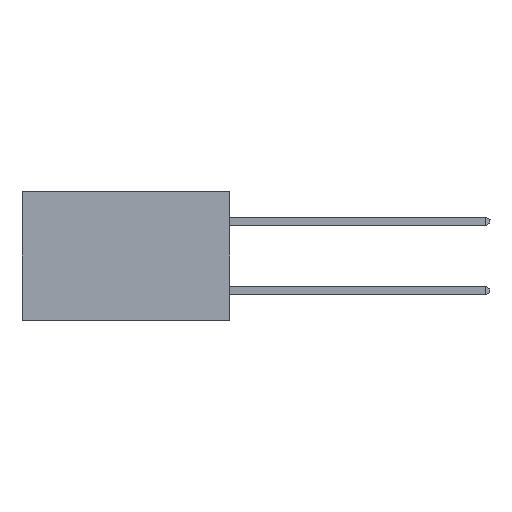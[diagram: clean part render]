
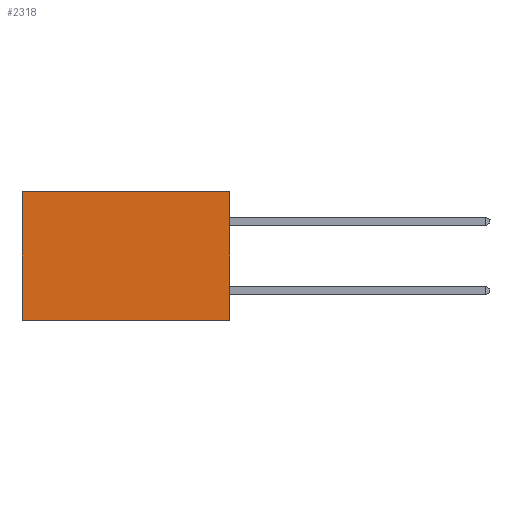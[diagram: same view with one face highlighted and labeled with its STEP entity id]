
A CAD part, left-side view. The second image highlights one B-rep face of the part: STEP entity #2318.
In plain terms, the highlighted planar face has unit normal (-1, 0, 0).
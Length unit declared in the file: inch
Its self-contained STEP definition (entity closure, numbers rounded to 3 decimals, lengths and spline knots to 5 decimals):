
#1065 = LINE ( 'NONE', #1849, #16956 ) ;
#1780 = EDGE_CURVE ( 'NONE', #18453, #9391, #6993, .T. ) ;
#1849 = CARTESIAN_POINT ( 'NONE',  ( 0.298, 0., 0. ) ) ;
#2318 = ADVANCED_FACE ( 'NONE', ( #10738 ), #8810, .F. ) ;
#3402 = CARTESIAN_POINT ( 'NONE',  ( 0.298, 0., 0. ) ) ;
#5031 = VECTOR ( 'NONE', #11629, 39.37008 ) ;
#5397 = EDGE_CURVE ( 'NONE', #8132, #18453, #1065, .T. ) ;
#5709 = CARTESIAN_POINT ( 'NONE',  ( 0.298, 0.6, -0.37 ) ) ;
#5795 = CARTESIAN_POINT ( 'NONE',  ( 0.298, 0., 0. ) ) ;
#6203 = ORIENTED_EDGE ( 'NONE', *, *, #12730, .T. ) ;
#6993 = LINE ( 'NONE', #11679, #11460 ) ;
#7573 = VERTEX_POINT ( 'NONE', #13256 ) ;
#7629 = ORIENTED_EDGE ( 'NONE', *, *, #1780, .F. ) ;
#7671 = DIRECTION ( 'NONE',  ( 0., 0., -1. ) ) ;
#8132 = VERTEX_POINT ( 'NONE', #3402 ) ;
#8725 = DIRECTION ( 'NONE',  ( 0., 1., 0. ) ) ;
#8810 = PLANE ( 'NONE',  #13599 ) ;
#9368 = DIRECTION ( 'NONE',  ( 0., 0., -1. ) ) ;
#9391 = VERTEX_POINT ( 'NONE', #5709 ) ;
#10480 = EDGE_CURVE ( 'NONE', #7573, #9391, #18217, .T. ) ;
#10492 = CARTESIAN_POINT ( 'NONE',  ( 0.298, 0., -0.37 ) ) ;
#10637 = CARTESIAN_POINT ( 'NONE',  ( 0.298, 0.6, 0. ) ) ;
#10738 = FACE_OUTER_BOUND ( 'NONE', #14293, .T. ) ;
#11450 = ORIENTED_EDGE ( 'NONE', *, *, #10480, .T. ) ;
#11460 = VECTOR ( 'NONE', #8725, 39.37008 ) ;
#11629 = DIRECTION ( 'NONE',  ( 0., 1., 0. ) ) ;
#11654 = ORIENTED_EDGE ( 'NONE', *, *, #5397, .F. ) ;
#11679 = CARTESIAN_POINT ( 'NONE',  ( 0.298, 0., -0.37 ) ) ;
#12730 = EDGE_CURVE ( 'NONE', #8132, #7573, #13474, .T. ) ;
#13256 = CARTESIAN_POINT ( 'NONE',  ( 0.298, 0.6, 0. ) ) ;
#13474 = LINE ( 'NONE', #17540, #5031 ) ;
#13599 = AXIS2_PLACEMENT_3D ( 'NONE', #5795, #16252, #17789 ) ;
#14242 = VECTOR ( 'NONE', #7671, 39.37008 ) ;
#14293 = EDGE_LOOP ( 'NONE', ( #11450, #7629, #11654, #6203 ) ) ;
#16252 = DIRECTION ( 'NONE',  ( 1., 0., 0. ) ) ;
#16956 = VECTOR ( 'NONE', #9368, 39.37008 ) ;
#17540 = CARTESIAN_POINT ( 'NONE',  ( 0.298, 0., 0. ) ) ;
#17789 = DIRECTION ( 'NONE',  ( 0., 0., -1. ) ) ;
#18217 = LINE ( 'NONE', #10637, #14242 ) ;
#18453 = VERTEX_POINT ( 'NONE', #10492 ) ;
